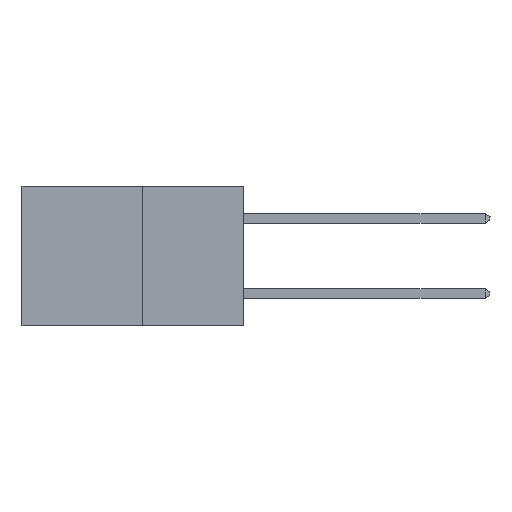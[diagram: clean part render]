
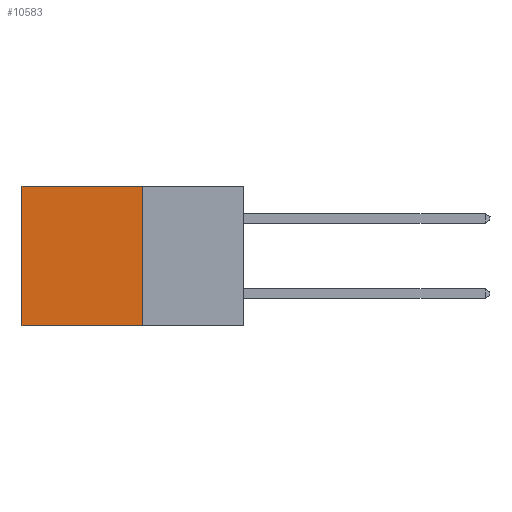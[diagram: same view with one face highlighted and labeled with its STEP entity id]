
A CAD part, left-side view. The second image highlights one B-rep face of the part: STEP entity #10583.
In plain terms, the highlighted planar face has unit normal (-1, 0, 0).
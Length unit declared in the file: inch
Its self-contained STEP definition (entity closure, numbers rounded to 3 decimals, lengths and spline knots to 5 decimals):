
#875 = CARTESIAN_POINT ( 'NONE',  ( 0.277, 0.59, 0. ) ) ;
#1088 = PLANE ( 'NONE',  #2566 ) ;
#1438 = ORIENTED_EDGE ( 'NONE', *, *, #2283, .T. ) ;
#1996 = EDGE_CURVE ( 'NONE', #13790, #4946, #3168, .T. ) ;
#2166 = VECTOR ( 'NONE', #11326, 39.37008 ) ;
#2283 = EDGE_CURVE ( 'NONE', #13790, #10728, #2437, .T. ) ;
#2437 = LINE ( 'NONE', #15534, #18261 ) ;
#2566 = AXIS2_PLACEMENT_3D ( 'NONE', #4108, #5639, #16413 ) ;
#2869 = CARTESIAN_POINT ( 'NONE',  ( 0.277, 0.59, -0.37 ) ) ;
#3168 = LINE ( 'NONE', #8190, #7203 ) ;
#3643 = CARTESIAN_POINT ( 'NONE',  ( 0.277, 0.27, -0.37 ) ) ;
#4108 = CARTESIAN_POINT ( 'NONE',  ( 0.277, 0.27, -0.37 ) ) ;
#4946 = VERTEX_POINT ( 'NONE', #15985 ) ;
#5086 = DIRECTION ( 'NONE',  ( 0., 0., -1. ) ) ;
#5343 = VECTOR ( 'NONE', #15128, 39.37008 ) ;
#5639 = DIRECTION ( 'NONE',  ( 1., 0., 0. ) ) ;
#6641 = ORIENTED_EDGE ( 'NONE', *, *, #14376, .T. ) ;
#7203 = VECTOR ( 'NONE', #5086, 39.37008 ) ;
#8190 = CARTESIAN_POINT ( 'NONE',  ( 0.277, 0.27, -0.37 ) ) ;
#10583 = ADVANCED_FACE ( 'NONE', ( #10895 ), #1088, .F. ) ;
#10728 = VERTEX_POINT ( 'NONE', #875 ) ;
#10895 = FACE_OUTER_BOUND ( 'NONE', #11572, .T. ) ;
#11326 = DIRECTION ( 'NONE',  ( 0., 1., 0. ) ) ;
#11572 = EDGE_LOOP ( 'NONE', ( #6641, #15312, #16758, #1438 ) ) ;
#13790 = VERTEX_POINT ( 'NONE', #16911 ) ;
#14037 = LINE ( 'NONE', #2869, #5343 ) ;
#14376 = EDGE_CURVE ( 'NONE', #10728, #16132, #14037, .T. ) ;
#15128 = DIRECTION ( 'NONE',  ( 0., 0., -1. ) ) ;
#15312 = ORIENTED_EDGE ( 'NONE', *, *, #17478, .F. ) ;
#15534 = CARTESIAN_POINT ( 'NONE',  ( 0.277, 0.27, 0. ) ) ;
#15607 = DIRECTION ( 'NONE',  ( 0., 1., 0. ) ) ;
#15985 = CARTESIAN_POINT ( 'NONE',  ( 0.277, 0.27, -0.37 ) ) ;
#16132 = VERTEX_POINT ( 'NONE', #19055 ) ;
#16413 = DIRECTION ( 'NONE',  ( 0., 0., -1. ) ) ;
#16758 = ORIENTED_EDGE ( 'NONE', *, *, #1996, .F. ) ;
#16911 = CARTESIAN_POINT ( 'NONE',  ( 0.277, 0.27, 0. ) ) ;
#17478 = EDGE_CURVE ( 'NONE', #4946, #16132, #17962, .T. ) ;
#17962 = LINE ( 'NONE', #3643, #2166 ) ;
#18261 = VECTOR ( 'NONE', #15607, 39.37008 ) ;
#19055 = CARTESIAN_POINT ( 'NONE',  ( 0.277, 0.59, -0.37 ) ) ;
